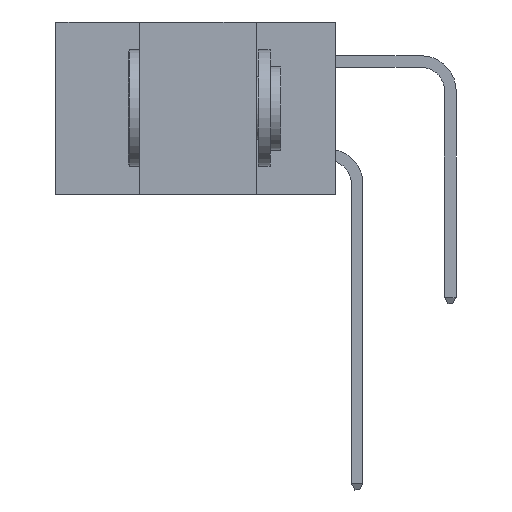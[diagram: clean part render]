
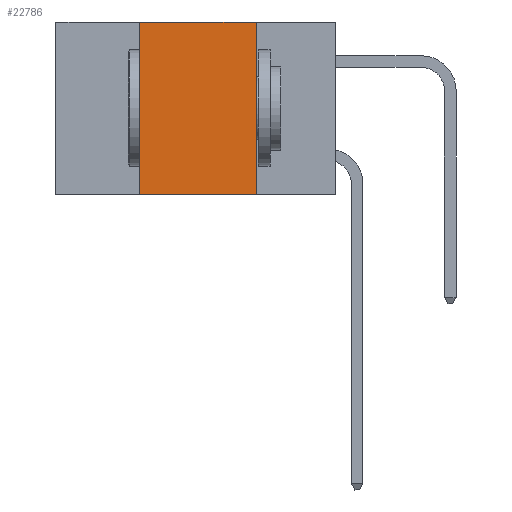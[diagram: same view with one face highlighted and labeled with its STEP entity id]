
A CAD part, left-side view. The second image highlights one B-rep face of the part: STEP entity #22786.
In plain terms, the highlighted planar face has unit normal (-1, 0, 0).
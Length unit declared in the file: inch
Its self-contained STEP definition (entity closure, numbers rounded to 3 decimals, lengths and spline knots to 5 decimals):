
#9 = FACE_OUTER_BOUND ( 'NONE', #16207, .T. ) ;
#60 = LINE ( 'NONE', #17255, #7757 ) ;
#113 = ORIENTED_EDGE ( 'NONE', *, *, #20857, .F. ) ;
#1827 = DIRECTION ( 'NONE',  ( 0., 0., -1. ) ) ;
#2465 = DIRECTION ( 'NONE',  ( 0., 0., -1. ) ) ;
#2838 = EDGE_CURVE ( 'NONE', #25548, #8386, #27655, .T. ) ;
#5340 = ORIENTED_EDGE ( 'NONE', *, *, #2838, .T. ) ;
#5429 = DIRECTION ( 'NONE',  ( 0., 0., 1. ) ) ;
#6531 = CARTESIAN_POINT ( 'NONE',  ( 0., 0.42, 0. ) ) ;
#7092 = VECTOR ( 'NONE', #13089, 39.37008 ) ;
#7554 = CARTESIAN_POINT ( 'NONE',  ( 0., 0.6, 0. ) ) ;
#7750 = CARTESIAN_POINT ( 'NONE',  ( 0., 0.6, 0. ) ) ;
#7757 = VECTOR ( 'NONE', #1827, 39.37008 ) ;
#8386 = VERTEX_POINT ( 'NONE', #31851 ) ;
#8492 = EDGE_CURVE ( 'NONE', #8788, #8386, #60, .T. ) ;
#8788 = VERTEX_POINT ( 'NONE', #15426 ) ;
#10340 = PLANE ( 'NONE',  #22322 ) ;
#10677 = CARTESIAN_POINT ( 'NONE',  ( 0., 0.6, -0.37 ) ) ;
#11341 = VECTOR ( 'NONE', #5429, 39.37008 ) ;
#12618 = VECTOR ( 'NONE', #30997, 39.37008 ) ;
#13089 = DIRECTION ( 'NONE',  ( 0., -1., 0. ) ) ;
#13714 = VERTEX_POINT ( 'NONE', #6531 ) ;
#15426 = CARTESIAN_POINT ( 'NONE',  ( 0., 0.17, 0. ) ) ;
#16207 = EDGE_LOOP ( 'NONE', ( #26348, #22154, #113, #5340 ) ) ;
#17255 = CARTESIAN_POINT ( 'NONE',  ( 0., 0.17, 0. ) ) ;
#18019 = DIRECTION ( 'NONE',  ( 1., 0., 0. ) ) ;
#18585 = LINE ( 'NONE', #20974, #11341 ) ;
#20857 = EDGE_CURVE ( 'NONE', #25548, #13714, #18585, .T. ) ;
#20974 = CARTESIAN_POINT ( 'NONE',  ( 0., 0.42, 0. ) ) ;
#22154 = ORIENTED_EDGE ( 'NONE', *, *, #29687, .F. ) ;
#22322 = AXIS2_PLACEMENT_3D ( 'NONE', #7554, #18019, #2465 ) ;
#22786 = ADVANCED_FACE ( 'NONE', ( #9 ), #10340, .F. ) ;
#25548 = VERTEX_POINT ( 'NONE', #26481 ) ;
#26348 = ORIENTED_EDGE ( 'NONE', *, *, #8492, .F. ) ;
#26481 = CARTESIAN_POINT ( 'NONE',  ( 0., 0.42, -0.37 ) ) ;
#27655 = LINE ( 'NONE', #10677, #7092 ) ;
#29687 = EDGE_CURVE ( 'NONE', #13714, #8788, #32388, .T. ) ;
#30997 = DIRECTION ( 'NONE',  ( 0., -1., 0. ) ) ;
#31851 = CARTESIAN_POINT ( 'NONE',  ( 0., 0.17, -0.37 ) ) ;
#32388 = LINE ( 'NONE', #7750, #12618 ) ;
